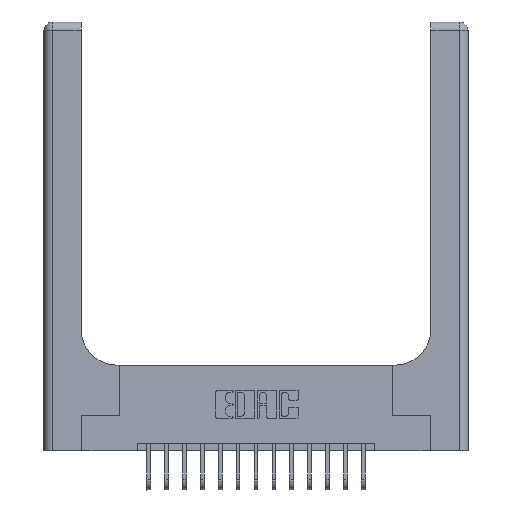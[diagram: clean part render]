
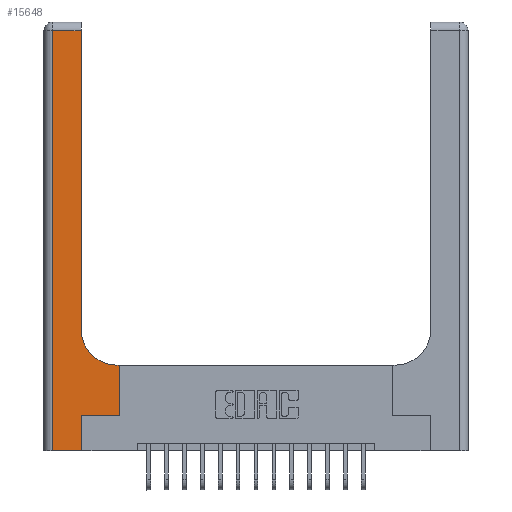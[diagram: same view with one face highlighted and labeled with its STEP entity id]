
A CAD part, top view. The second image highlights one B-rep face of the part: STEP entity #15648.
In plain terms, the highlighted planar face has unit normal (0, 0, 1).
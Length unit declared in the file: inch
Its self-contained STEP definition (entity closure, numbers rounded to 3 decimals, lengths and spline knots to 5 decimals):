
#271 = EDGE_CURVE ( 'NONE', #16160, #7062, #14238, .T. ) ;
#304 = VERTEX_POINT ( 'NONE', #3609 ) ;
#317 = CARTESIAN_POINT ( 'NONE',  ( 0.51, 0.6, 0.37 ) ) ;
#504 = VERTEX_POINT ( 'NONE', #13321 ) ;
#1074 = CARTESIAN_POINT ( 'NONE',  ( 0.528, 0.25, 0.37 ) ) ;
#1223 = ORIENTED_EDGE ( 'NONE', *, *, #13383, .T. ) ;
#1281 = CARTESIAN_POINT ( 'NONE',  ( 0.265, 0., 0.37 ) ) ;
#1354 = LINE ( 'NONE', #12190, #18621 ) ;
#1712 = DIRECTION ( 'NONE',  ( 0., 0., -1. ) ) ;
#1716 = CARTESIAN_POINT ( 'NONE',  ( 0.265, 0.25, 0.37 ) ) ;
#1828 = CARTESIAN_POINT ( 'NONE',  ( 0.06, 2.94, 0.37 ) ) ;
#3590 = VERTEX_POINT ( 'NONE', #1281 ) ;
#3609 = CARTESIAN_POINT ( 'NONE',  ( 0.528, 0.6, 0.37 ) ) ;
#3991 = ORIENTED_EDGE ( 'NONE', *, *, #18523, .T. ) ;
#4304 = VECTOR ( 'NONE', #11856, 39.37008 ) ;
#4325 = LINE ( 'NONE', #4521, #4304 ) ;
#4495 = CARTESIAN_POINT ( 'NONE',  ( 0.26, 2.94, 0.37 ) ) ;
#4521 = CARTESIAN_POINT ( 'NONE',  ( 0., 0., 0.37 ) ) ;
#5023 = EDGE_LOOP ( 'NONE', ( #6868, #6759, #5980, #11909, #12230, #3991, #8232, #1223, #11926 ) ) ;
#5586 = LINE ( 'NONE', #7295, #19047 ) ;
#5738 = CARTESIAN_POINT ( 'NONE',  ( 0.265, 0.25, 0.37 ) ) ;
#5865 = DIRECTION ( 'NONE',  ( 0., 1., 0. ) ) ;
#5980 = ORIENTED_EDGE ( 'NONE', *, *, #6442, .T. ) ;
#6025 = PLANE ( 'NONE',  #14863 ) ;
#6442 = EDGE_CURVE ( 'NONE', #7062, #504, #7782, .T. ) ;
#6759 = ORIENTED_EDGE ( 'NONE', *, *, #271, .T. ) ;
#6868 = ORIENTED_EDGE ( 'NONE', *, *, #13517, .T. ) ;
#6879 = EDGE_CURVE ( 'NONE', #8449, #17945, #7748, .T. ) ;
#7062 = VERTEX_POINT ( 'NONE', #1828 ) ;
#7295 = CARTESIAN_POINT ( 'NONE',  ( 0.265, 0., 0.37 ) ) ;
#7421 = VECTOR ( 'NONE', #17831, 39.37008 ) ;
#7748 = CIRCLE ( 'NONE', #19571, 0.25 ) ;
#7782 = LINE ( 'NONE', #13884, #7421 ) ;
#8232 = ORIENTED_EDGE ( 'NONE', *, *, #16383, .T. ) ;
#8449 = VERTEX_POINT ( 'NONE', #317 ) ;
#8456 = VECTOR ( 'NONE', #16004, 39.37008 ) ;
#8581 = DIRECTION ( 'NONE',  ( -1., 0., 0. ) ) ;
#8890 = LINE ( 'NONE', #17903, #17017 ) ;
#9261 = FACE_OUTER_BOUND ( 'NONE', #5023, .T. ) ;
#9287 = VERTEX_POINT ( 'NONE', #16276 ) ;
#10012 = DIRECTION ( 'NONE',  ( 0., 1., 0. ) ) ;
#10197 = CARTESIAN_POINT ( 'NONE',  ( 0.26, 0.85, 0.37 ) ) ;
#11856 = DIRECTION ( 'NONE',  ( 1., 0., 0. ) ) ;
#11909 = ORIENTED_EDGE ( 'NONE', *, *, #17112, .T. ) ;
#11926 = ORIENTED_EDGE ( 'NONE', *, *, #6879, .T. ) ;
#12168 = VECTOR ( 'NONE', #17343, 39.37008 ) ;
#12190 = CARTESIAN_POINT ( 'NONE',  ( 0.26, 3., 0.37 ) ) ;
#12230 = ORIENTED_EDGE ( 'NONE', *, *, #17359, .T. ) ;
#12923 = CARTESIAN_POINT ( 'NONE',  ( 0., 2.94, 0.37 ) ) ;
#13321 = CARTESIAN_POINT ( 'NONE',  ( 0.06, 0., 0.37 ) ) ;
#13383 = EDGE_CURVE ( 'NONE', #304, #8449, #8890, .T. ) ;
#13517 = EDGE_CURVE ( 'NONE', #17945, #16160, #1354, .T. ) ;
#13750 = LINE ( 'NONE', #5738, #14603 ) ;
#13759 = CARTESIAN_POINT ( 'NONE',  ( 0.51, 0.85, 0.37 ) ) ;
#13884 = CARTESIAN_POINT ( 'NONE',  ( 0.06, 3., 0.37 ) ) ;
#14238 = LINE ( 'NONE', #12923, #12168 ) ;
#14603 = VECTOR ( 'NONE', #17971, 39.37008 ) ;
#14863 = AXIS2_PLACEMENT_3D ( 'NONE', #15532, #1712, #18256 ) ;
#14976 = DIRECTION ( 'NONE',  ( 1., 0., 0. ) ) ;
#15532 = CARTESIAN_POINT ( 'NONE',  ( 0., 3., 0.37 ) ) ;
#15648 = ADVANCED_FACE ( 'NONE', ( #9261 ), #6025, .F. ) ;
#16004 = DIRECTION ( 'NONE',  ( 0., 1., 0. ) ) ;
#16160 = VERTEX_POINT ( 'NONE', #4495 ) ;
#16276 = CARTESIAN_POINT ( 'NONE',  ( 0.528, 0.25, 0.37 ) ) ;
#16383 = EDGE_CURVE ( 'NONE', #9287, #304, #19212, .T. ) ;
#17017 = VECTOR ( 'NONE', #8581, 39.37008 ) ;
#17112 = EDGE_CURVE ( 'NONE', #504, #3590, #4325, .T. ) ;
#17293 = VERTEX_POINT ( 'NONE', #1716 ) ;
#17343 = DIRECTION ( 'NONE',  ( -1., 0., 0. ) ) ;
#17359 = EDGE_CURVE ( 'NONE', #3590, #17293, #5586, .T. ) ;
#17831 = DIRECTION ( 'NONE',  ( 0., -1., 0. ) ) ;
#17903 = CARTESIAN_POINT ( 'NONE',  ( 0.26, 0.6, 0.37 ) ) ;
#17945 = VERTEX_POINT ( 'NONE', #10197 ) ;
#17971 = DIRECTION ( 'NONE',  ( 1., 0., 0. ) ) ;
#18185 = DIRECTION ( 'NONE',  ( 0., 0., -1. ) ) ;
#18256 = DIRECTION ( 'NONE',  ( -1., 0., 0. ) ) ;
#18523 = EDGE_CURVE ( 'NONE', #17293, #9287, #13750, .T. ) ;
#18621 = VECTOR ( 'NONE', #5865, 39.37008 ) ;
#19047 = VECTOR ( 'NONE', #10012, 39.37008 ) ;
#19212 = LINE ( 'NONE', #1074, #8456 ) ;
#19571 = AXIS2_PLACEMENT_3D ( 'NONE', #13759, #18185, #14976 ) ;
